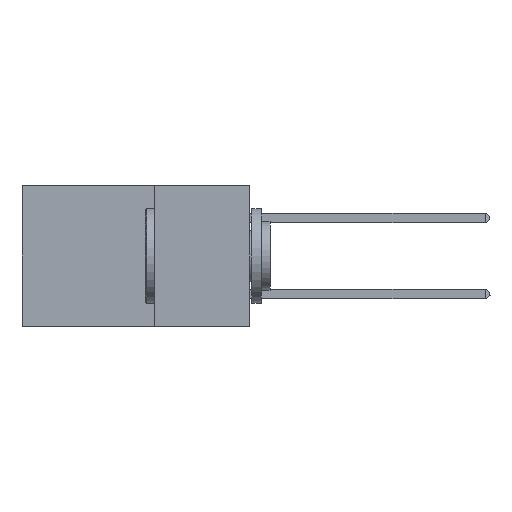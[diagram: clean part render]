
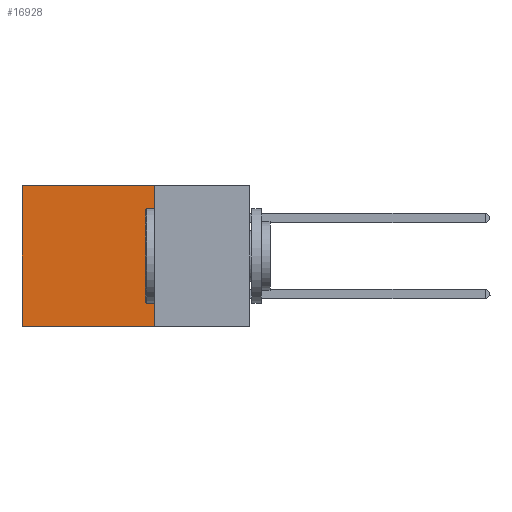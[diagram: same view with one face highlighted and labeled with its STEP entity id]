
A CAD part, left-side view. The second image highlights one B-rep face of the part: STEP entity #16928.
In plain terms, the highlighted planar face has unit normal (-1, 0, 0).
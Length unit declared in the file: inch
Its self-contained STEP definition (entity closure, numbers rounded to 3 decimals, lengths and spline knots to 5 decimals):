
#163 = VECTOR ( 'NONE', #9418, 39.37008 ) ;
#380 = EDGE_CURVE ( 'NONE', #4887, #10643, #753, .T. ) ;
#526 = ORIENTED_EDGE ( 'NONE', *, *, #1201, .F. ) ;
#753 = LINE ( 'NONE', #9668, #7150 ) ;
#1201 = EDGE_CURVE ( 'NONE', #7746, #10643, #7365, .T. ) ;
#1585 = DIRECTION ( 'NONE',  ( 0., 0., -1. ) ) ;
#2349 = CARTESIAN_POINT ( 'NONE',  ( 0.2875, 0.25, 0. ) ) ;
#2412 = EDGE_CURVE ( 'NONE', #15798, #7746, #3469, .T. ) ;
#2485 = CARTESIAN_POINT ( 'NONE',  ( 0.2875, 0.25, 0. ) ) ;
#2625 = CARTESIAN_POINT ( 'NONE',  ( 0.2875, 0.25, 0. ) ) ;
#2935 = EDGE_LOOP ( 'NONE', ( #15400, #526, #17381, #14345 ) ) ;
#2979 = CARTESIAN_POINT ( 'NONE',  ( 0.2875, 0.6, 0. ) ) ;
#3469 = LINE ( 'NONE', #2625, #12919 ) ;
#3750 = AXIS2_PLACEMENT_3D ( 'NONE', #14200, #10111, #15428 ) ;
#3792 = DIRECTION ( 'NONE',  ( 0., 0., -1. ) ) ;
#3861 = CARTESIAN_POINT ( 'NONE',  ( 0.2875, 0.25, -0.37 ) ) ;
#4887 = VERTEX_POINT ( 'NONE', #2979 ) ;
#5162 = DIRECTION ( 'NONE',  ( 0., 1., 0. ) ) ;
#7150 = VECTOR ( 'NONE', #1585, 39.37008 ) ;
#7365 = LINE ( 'NONE', #3861, #163 ) ;
#7746 = VERTEX_POINT ( 'NONE', #9539 ) ;
#9418 = DIRECTION ( 'NONE',  ( 0., 1., 0. ) ) ;
#9539 = CARTESIAN_POINT ( 'NONE',  ( 0.2875, 0.25, -0.37 ) ) ;
#9668 = CARTESIAN_POINT ( 'NONE',  ( 0.2875, 0.6, 0. ) ) ;
#10111 = DIRECTION ( 'NONE',  ( 1., 0., 0. ) ) ;
#10643 = VERTEX_POINT ( 'NONE', #13963 ) ;
#11786 = LINE ( 'NONE', #2485, #16809 ) ;
#12703 = EDGE_CURVE ( 'NONE', #15798, #4887, #11786, .T. ) ;
#12919 = VECTOR ( 'NONE', #3792, 39.37008 ) ;
#13963 = CARTESIAN_POINT ( 'NONE',  ( 0.2875, 0.6, -0.37 ) ) ;
#14200 = CARTESIAN_POINT ( 'NONE',  ( 0.2875, 0.25, 0. ) ) ;
#14345 = ORIENTED_EDGE ( 'NONE', *, *, #12703, .T. ) ;
#14990 = FACE_OUTER_BOUND ( 'NONE', #2935, .T. ) ;
#15400 = ORIENTED_EDGE ( 'NONE', *, *, #380, .T. ) ;
#15428 = DIRECTION ( 'NONE',  ( 0., 0., -1. ) ) ;
#15595 = PLANE ( 'NONE',  #3750 ) ;
#15798 = VERTEX_POINT ( 'NONE', #2349 ) ;
#16809 = VECTOR ( 'NONE', #5162, 39.37008 ) ;
#16928 = ADVANCED_FACE ( 'NONE', ( #14990 ), #15595, .F. ) ;
#17381 = ORIENTED_EDGE ( 'NONE', *, *, #2412, .F. ) ;
